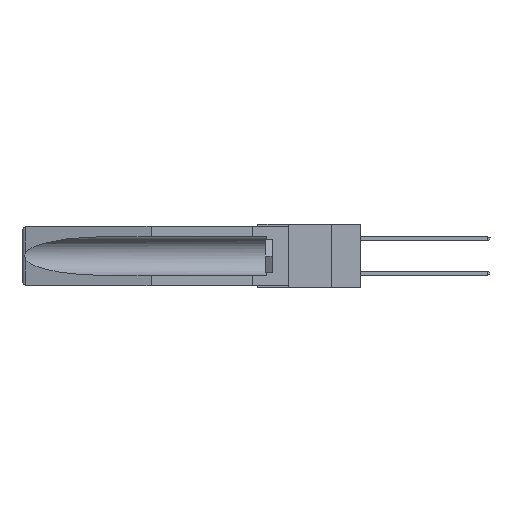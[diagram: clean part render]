
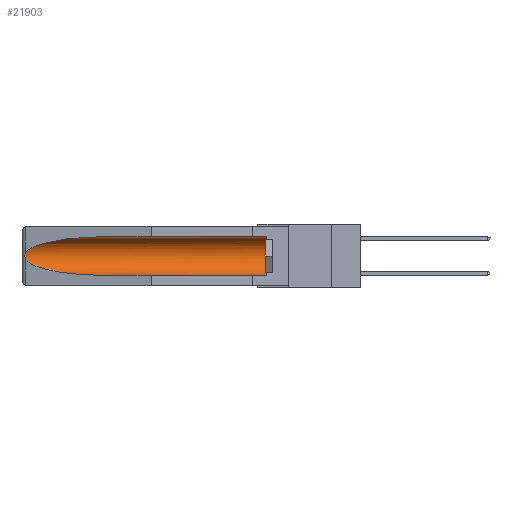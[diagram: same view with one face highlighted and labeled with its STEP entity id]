
A CAD part, left-side view. The second image highlights one B-rep face of the part: STEP entity #21903.
In plain terms, the highlighted cylindrical face has radius 2.857 mm (diameter 5.715 mm), a partial arc.
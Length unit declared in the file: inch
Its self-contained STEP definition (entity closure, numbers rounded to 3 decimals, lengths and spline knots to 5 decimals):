
#1181 = CARTESIAN_POINT ( 'NONE',  ( 0.155, 0.126, -0.059 ) ) ;
#1226 = ORIENTED_EDGE ( 'NONE', *, *, #17813, .T. ) ;
#1507 = CARTESIAN_POINT ( 'NONE',  ( 0.26537, 1.52718, -0.14972 ) ) ;
#1597 = ORIENTED_EDGE ( 'NONE', *, *, #8964, .T. ) ;
#1873 = CARTESIAN_POINT ( 'NONE',  ( 0.2675, 1.53308, -0.17534 ) ) ;
#1977 = CARTESIAN_POINT ( 'NONE',  ( 0.26537, 1.52718, -0.19328 ) ) ;
#2808 = CARTESIAN_POINT ( 'NONE',  ( 0.26537, 1.52718, -0.19328 ) ) ;
#3253 = CARTESIAN_POINT ( 'NONE',  ( 0.155, 1.07973, -0.284 ) ) ;
#3388 = VECTOR ( 'NONE', #14580, 39.37008 ) ;
#3690 =( BOUNDED_CURVE ( )  B_SPLINE_CURVE ( 3, ( #2808, #5627, #18667, #3253 ),
 .UNSPECIFIED., .F., .F. ) 
 B_SPLINE_CURVE_WITH_KNOTS ( ( 4, 4 ),
 ( 0.1948, 1.5708 ),
 .UNSPECIFIED. ) 
 CURVE ( )  GEOMETRIC_REPRESENTATION_ITEM ( )  RATIONAL_B_SPLINE_CURVE ( ( 1., 0.848, 0.848, 1. ) ) 
 REPRESENTATION_ITEM ( '' )  );
#4079 = VERTEX_POINT ( 'NONE', #1181 ) ;
#4144 = CARTESIAN_POINT ( 'NONE',  ( 0.26597, 1.52961, -0.15275 ) ) ;
#5013 = EDGE_CURVE ( 'NONE', #4079, #26898, #10242, .T. ) ;
#5111 = CARTESIAN_POINT ( 'NONE',  ( 0.155, -0.30754, -0.284 ) ) ;
#5126 = EDGE_CURVE ( 'NONE', #26898, #25328, #11542, .T. ) ;
#5157 = CARTESIAN_POINT ( 'NONE',  ( 0.155, 1.07973, -0.284 ) ) ;
#5430 = VERTEX_POINT ( 'NONE', #11710 ) ;
#5627 = CARTESIAN_POINT ( 'NONE',  ( 0.25451, 1.48313, -0.24835 ) ) ;
#6857 = CARTESIAN_POINT ( 'NONE',  ( 0.26654, 1.53092, -0.15636 ) ) ;
#8393 = CIRCLE ( 'NONE', #20772, 0.1125 ) ;
#8539 = CYLINDRICAL_SURFACE ( 'NONE', #16482, 0.1125 ) ;
#8964 = EDGE_CURVE ( 'NONE', #14909, #4079, #8393, .T. ) ;
#10242 = LINE ( 'NONE', #32130, #3388 ) ;
#11542 =( BOUNDED_CURVE ( )  B_SPLINE_CURVE ( 3, ( #29696, #24776, #32468, #1507 ),
 .UNSPECIFIED., .F., .T. ) 
 B_SPLINE_CURVE_WITH_KNOTS ( ( 4, 4 ),
 ( 4.71239, 6.08839 ),
 .UNSPECIFIED. ) 
 CURVE ( )  GEOMETRIC_REPRESENTATION_ITEM ( )  RATIONAL_B_SPLINE_CURVE ( ( 1., 0.848, 0.848, 1. ) ) 
 REPRESENTATION_ITEM ( '' )  );
#11710 = CARTESIAN_POINT ( 'NONE',  ( 0.26537, 1.52718, -0.19328 ) ) ;
#12340 = CARTESIAN_POINT ( 'NONE',  ( 0.26537, 1.52718, -0.14972 ) ) ;
#12418 = DIRECTION ( 'NONE',  ( 0., 0., 1. ) ) ;
#12455 = VECTOR ( 'NONE', #26497, 39.37008 ) ;
#14495 = CARTESIAN_POINT ( 'NONE',  ( 0.2675, 1.53308, -0.16763 ) ) ;
#14578 = FACE_OUTER_BOUND ( 'NONE', #24697, .T. ) ;
#14580 = DIRECTION ( 'NONE',  ( 0., 1., 0. ) ) ;
#14617 = CARTESIAN_POINT ( 'NONE',  ( 0.26655, 1.53094, -0.18657 ) ) ;
#14909 = VERTEX_POINT ( 'NONE', #28640 ) ;
#15157 = EDGE_CURVE ( 'NONE', #25328, #5430, #26955, .T. ) ;
#15772 = CARTESIAN_POINT ( 'NONE',  ( 0.155, 1.07973, -0.059 ) ) ;
#16482 = AXIS2_PLACEMENT_3D ( 'NONE', #25424, #20144, #12418 ) ;
#17083 = CARTESIAN_POINT ( 'NONE',  ( 0.2673, 1.53269, -0.17917 ) ) ;
#17813 = EDGE_CURVE ( 'NONE', #5430, #22116, #3690, .T. ) ;
#18667 = CARTESIAN_POINT ( 'NONE',  ( 0.21114, 1.30732, -0.284 ) ) ;
#19038 = CARTESIAN_POINT ( 'NONE',  ( 0.26537, 1.52718, -0.14972 ) ) ;
#20144 = DIRECTION ( 'NONE',  ( 0., 1., 0. ) ) ;
#20772 = AXIS2_PLACEMENT_3D ( 'NONE', #27653, #27768, #30446 ) ;
#21271 = ORIENTED_EDGE ( 'NONE', *, *, #15157, .T. ) ;
#21728 = ORIENTED_EDGE ( 'NONE', *, *, #5126, .T. ) ;
#21903 = ADVANCED_FACE ( 'NONE', ( #14578 ), #8539, .F. ) ;
#22116 = VERTEX_POINT ( 'NONE', #5157 ) ;
#22929 = ORIENTED_EDGE ( 'NONE', *, *, #23366, .F. ) ;
#23366 = EDGE_CURVE ( 'NONE', #14909, #22116, #30900, .T. ) ;
#24697 = EDGE_LOOP ( 'NONE', ( #21728, #21271, #1226, #22929, #1597, #31520 ) ) ;
#24776 = CARTESIAN_POINT ( 'NONE',  ( 0.21114, 1.30732, -0.059 ) ) ;
#24909 = CARTESIAN_POINT ( 'NONE',  ( 0.26597, 1.5296, -0.19026 ) ) ;
#25018 = CARTESIAN_POINT ( 'NONE',  ( 0.2673, 1.5327, -0.16383 ) ) ;
#25328 = VERTEX_POINT ( 'NONE', #19038 ) ;
#25424 = CARTESIAN_POINT ( 'NONE',  ( 0.155, -0.30754, -0.1715 ) ) ;
#26497 = DIRECTION ( 'NONE',  ( 0., 1., 0. ) ) ;
#26898 = VERTEX_POINT ( 'NONE', #15772 ) ;
#26955 = B_SPLINE_CURVE_WITH_KNOTS ( 'NONE', 3,
 ( #12340, #4144, #6857, #25018, #14495, #1873, #17083, #14617, #24909, #1977 ),
 .UNSPECIFIED., .F., .F.,
 ( 4, 2, 2, 2, 4 ),
 ( 0., 0.00029, 0.00058, 0.00087, 0.00117 ),
 .UNSPECIFIED. ) ;
#27653 = CARTESIAN_POINT ( 'NONE',  ( 0.155, 0.126, -0.1715 ) ) ;
#27768 = DIRECTION ( 'NONE',  ( 0., -1., 0. ) ) ;
#28640 = CARTESIAN_POINT ( 'NONE',  ( 0.155, 0.126, -0.284 ) ) ;
#29696 = CARTESIAN_POINT ( 'NONE',  ( 0.155, 1.07973, -0.059 ) ) ;
#30446 = DIRECTION ( 'NONE',  ( 0., 0., 1. ) ) ;
#30900 = LINE ( 'NONE', #5111, #12455 ) ;
#31520 = ORIENTED_EDGE ( 'NONE', *, *, #5013, .T. ) ;
#32130 = CARTESIAN_POINT ( 'NONE',  ( 0.155, -0.30754, -0.059 ) ) ;
#32468 = CARTESIAN_POINT ( 'NONE',  ( 0.25451, 1.48313, -0.09465 ) ) ;
